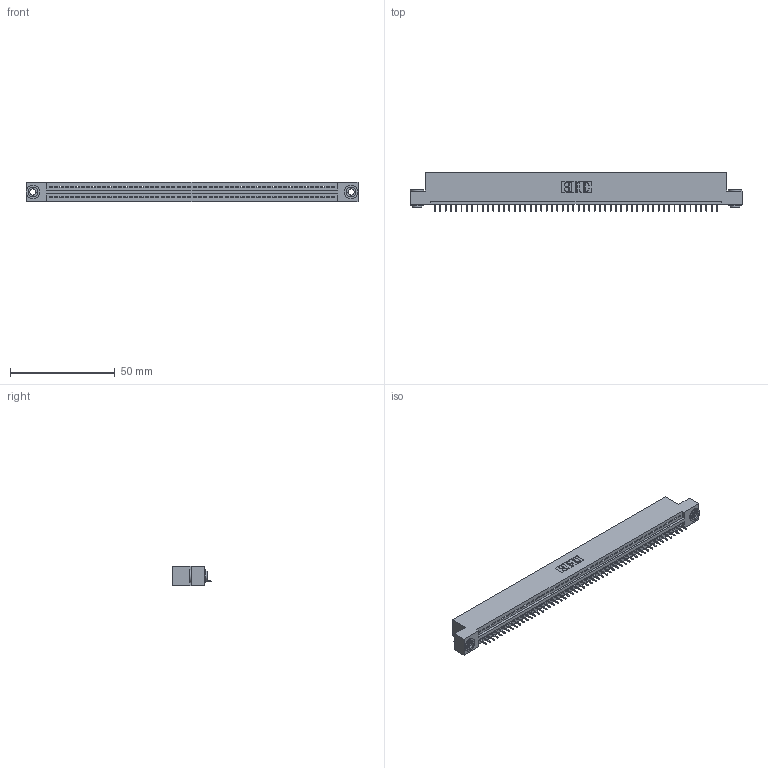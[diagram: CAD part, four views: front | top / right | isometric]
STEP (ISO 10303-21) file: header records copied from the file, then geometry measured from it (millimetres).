
FILE_DESCRIPTION (( 'STEP AP203' ), '1' );
FILE_NAME ('895-054-525-103.STEP', '2020-09-27T13:52:58', ( '' ), ( '' ), 'SwSTEP 2.0', 'SolidWorks 2020', '' );
FILE_SCHEMA (( 'CONFIG_CONTROL_DESIGN' ));
Length unit declared in the file: inch
Products named in the file (4): 345-250-002_345-250-002-102; 845 Part_Flush Mounting Lugs - 0.156 Dia-TH; 895-054-525-103; 345-292-001_345-293-125
Assembly tree (57 placements, depth 2):
  895-054-525-103
    845 Part_Flush Mounting Lugs - 0.156 Dia-TH
    345-292-001_345-293-125  x54
    345-250-002_345-250-002-102  x2
Bounding box: 158.37 x 18.72 x 9.4 mm (x, y, z)
Volume: 14939.3 mm3; surface area: 19495.3 mm2
Topology: 57 solids, 57 shells, 3512 faces, 10137 edges, 6538 vertices
Faces by surface type: plane 2574, cylinder 930, cone 8
Entity records: 39750 total; most frequent: CARTESIAN_POINT 6861, ORIENTED_EDGE 6842, DIRECTION 6007, EDGE_CURVE 3421, VECTOR 3053, LINE 3053, VERTEX_POINT 2274, AXIS2_PLACEMENT_3D 1477
